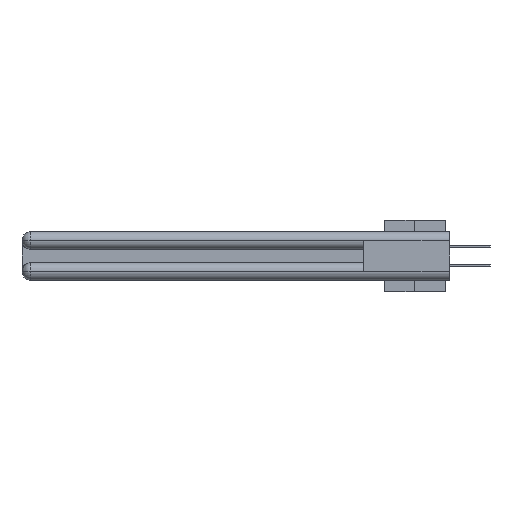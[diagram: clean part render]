
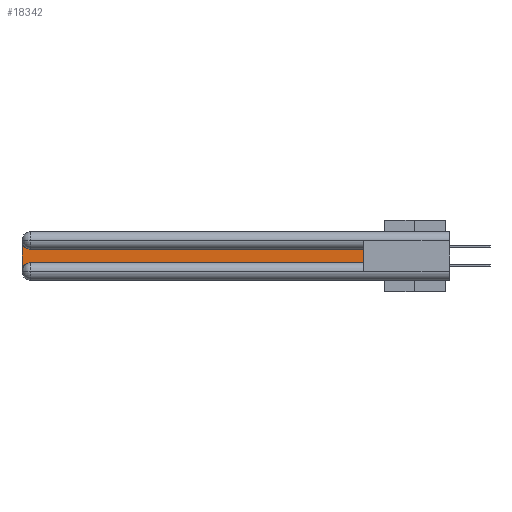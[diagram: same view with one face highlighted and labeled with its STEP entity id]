
A CAD part, left-side view. The second image highlights one B-rep face of the part: STEP entity #18342.
In plain terms, the highlighted planar face has unit normal (-1, 0, 0).
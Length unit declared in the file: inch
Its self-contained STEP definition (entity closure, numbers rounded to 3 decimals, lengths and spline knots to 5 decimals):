
#428 = LINE ( 'NONE', #30975, #2963 ) ;
#1309 = ORIENTED_EDGE ( 'NONE', *, *, #22422, .T. ) ;
#1981 = ORIENTED_EDGE ( 'NONE', *, *, #32614, .T. ) ;
#2963 = VECTOR ( 'NONE', #40458, 39.37008 ) ;
#3745 = ORIENTED_EDGE ( 'NONE', *, *, #13090, .T. ) ;
#4337 = DIRECTION ( 'NONE',  ( 0., 0., -1. ) ) ;
#4874 = ORIENTED_EDGE ( 'NONE', *, *, #31725, .T. ) ;
#5144 = EDGE_CURVE ( 'NONE', #16265, #7588, #31542, .T. ) ;
#6929 = AXIS2_PLACEMENT_3D ( 'NONE', #26165, #39276, #7428 ) ;
#7284 = DIRECTION ( 'NONE',  ( 1., 0., 0. ) ) ;
#7417 = PLANE ( 'NONE',  #41317 ) ;
#7428 = DIRECTION ( 'NONE',  ( 0., 0., -1. ) ) ;
#7588 = VERTEX_POINT ( 'NONE', #16920 ) ;
#8077 = LINE ( 'NONE', #21473, #30555 ) ;
#9541 = DIRECTION ( 'NONE',  ( 0., 0., -1. ) ) ;
#10588 = CARTESIAN_POINT ( 'NONE',  ( 0.075, 0.6, -0.2175 ) ) ;
#10996 = ORIENTED_EDGE ( 'NONE', *, *, #36405, .T. ) ;
#12709 = LINE ( 'NONE', #37124, #28690 ) ;
#12725 = EDGE_LOOP ( 'NONE', ( #10996, #1981, #1309, #36174, #3745, #4874 ) ) ;
#12948 = VERTEX_POINT ( 'NONE', #10588 ) ;
#13090 = EDGE_CURVE ( 'NONE', #7588, #12948, #8077, .T. ) ;
#13176 = CARTESIAN_POINT ( 'NONE',  ( 0.075, 2.94, -0.0625 ) ) ;
#13791 = CARTESIAN_POINT ( 'NONE',  ( 0.075, 3., -0.2775 ) ) ;
#13823 = CARTESIAN_POINT ( 'NONE',  ( 0.075, 3., -0.1225 ) ) ;
#16265 = VERTEX_POINT ( 'NONE', #13791 ) ;
#16920 = CARTESIAN_POINT ( 'NONE',  ( 0.075, 2.94, -0.2175 ) ) ;
#17471 = CARTESIAN_POINT ( 'NONE',  ( 0.075, 0.6, -0.1225 ) ) ;
#18342 = ADVANCED_FACE ( 'NONE', ( #31029 ), #7417, .F. ) ;
#20675 = CARTESIAN_POINT ( 'NONE',  ( 0.075, 0.6, -0.1225 ) ) ;
#21473 = CARTESIAN_POINT ( 'NONE',  ( 0.075, 0.6, -0.2175 ) ) ;
#21727 = LINE ( 'NONE', #20675, #26240 ) ;
#22422 = EDGE_CURVE ( 'NONE', #27597, #16265, #428, .T. ) ;
#23234 = CARTESIAN_POINT ( 'NONE',  ( 0.075, 2.94, -0.1225 ) ) ;
#26165 = CARTESIAN_POINT ( 'NONE',  ( 0.075, 2.94, -0.2775 ) ) ;
#26240 = VECTOR ( 'NONE', #27649, 39.37008 ) ;
#27597 = VERTEX_POINT ( 'NONE', #41215 ) ;
#27649 = DIRECTION ( 'NONE',  ( 0., 1., 0. ) ) ;
#27892 = VERTEX_POINT ( 'NONE', #17471 ) ;
#28690 = VECTOR ( 'NONE', #40344, 39.37008 ) ;
#30555 = VECTOR ( 'NONE', #30984, 39.37008 ) ;
#30975 = CARTESIAN_POINT ( 'NONE',  ( 0.075, 3., -0.2175 ) ) ;
#30984 = DIRECTION ( 'NONE',  ( 0., -1., 0. ) ) ;
#31029 = FACE_OUTER_BOUND ( 'NONE', #12725, .T. ) ;
#31542 = CIRCLE ( 'NONE', #6929, 0.06 ) ;
#31725 = EDGE_CURVE ( 'NONE', #12948, #27892, #12709, .T. ) ;
#32614 = EDGE_CURVE ( 'NONE', #39973, #27597, #33692, .T. ) ;
#33692 = CIRCLE ( 'NONE', #40877, 0.06 ) ;
#35526 = DIRECTION ( 'NONE',  ( 1., 0., 0. ) ) ;
#36174 = ORIENTED_EDGE ( 'NONE', *, *, #5144, .T. ) ;
#36405 = EDGE_CURVE ( 'NONE', #27892, #39973, #21727, .T. ) ;
#37124 = CARTESIAN_POINT ( 'NONE',  ( 0.075, 0.6, -0.2175 ) ) ;
#39276 = DIRECTION ( 'NONE',  ( 1., 0., 0. ) ) ;
#39973 = VERTEX_POINT ( 'NONE', #23234 ) ;
#40344 = DIRECTION ( 'NONE',  ( 0., 0., 1. ) ) ;
#40458 = DIRECTION ( 'NONE',  ( 0., 0., -1. ) ) ;
#40877 = AXIS2_PLACEMENT_3D ( 'NONE', #13176, #35526, #9541 ) ;
#41215 = CARTESIAN_POINT ( 'NONE',  ( 0.075, 3., -0.0625 ) ) ;
#41317 = AXIS2_PLACEMENT_3D ( 'NONE', #13823, #7284, #4337 ) ;
